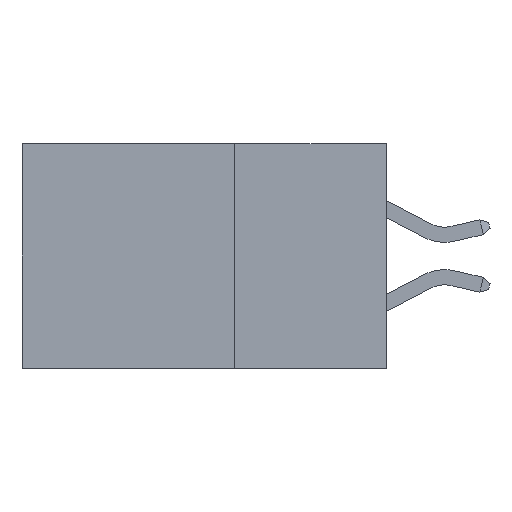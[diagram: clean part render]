
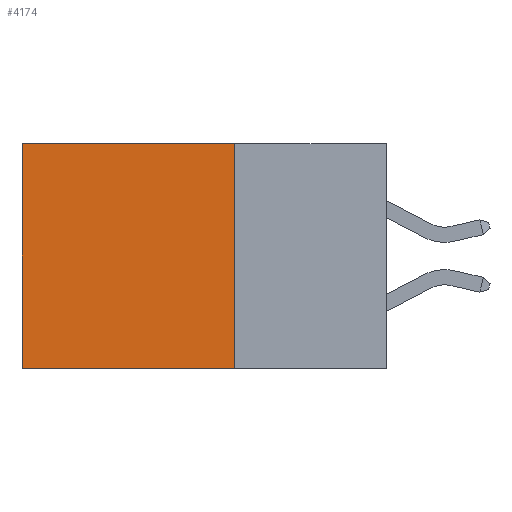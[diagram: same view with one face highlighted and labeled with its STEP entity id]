
A CAD part, left-side view. The second image highlights one B-rep face of the part: STEP entity #4174.
In plain terms, the highlighted planar face has unit normal (-1, 0, 0).
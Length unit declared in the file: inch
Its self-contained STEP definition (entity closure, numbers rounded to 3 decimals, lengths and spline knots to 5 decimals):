
#1862 = DIRECTION ( 'NONE',  ( 0., 0., -1. ) ) ;
#2205 = DIRECTION ( 'NONE',  ( 0., 1., 0. ) ) ;
#2445 = PLANE ( 'NONE',  #5829 ) ;
#2631 = LINE ( 'NONE', #12077, #5681 ) ;
#2814 = DIRECTION ( 'NONE',  ( 0., 0., -1. ) ) ;
#3792 = LINE ( 'NONE', #11962, #10301 ) ;
#4174 = ADVANCED_FACE ( 'NONE', ( #11785 ), #2445, .F. ) ;
#4543 = VECTOR ( 'NONE', #5913, 39.37008 ) ;
#4749 = DIRECTION ( 'NONE',  ( 0., 0., -1. ) ) ;
#5252 = ORIENTED_EDGE ( 'NONE', *, *, #10076, .T. ) ;
#5388 = CARTESIAN_POINT ( 'NONE',  ( 0.298, 0.25, -0.37 ) ) ;
#5681 = VECTOR ( 'NONE', #4749, 39.37008 ) ;
#5691 = LINE ( 'NONE', #14595, #4543 ) ;
#5829 = AXIS2_PLACEMENT_3D ( 'NONE', #8624, #8893, #2814 ) ;
#5913 = DIRECTION ( 'NONE',  ( 0., 1., 0. ) ) ;
#6825 = CARTESIAN_POINT ( 'NONE',  ( 0.298, 0.6, 0. ) ) ;
#7358 = ORIENTED_EDGE ( 'NONE', *, *, #8636, .F. ) ;
#7545 = VERTEX_POINT ( 'NONE', #5388 ) ;
#8370 = EDGE_CURVE ( 'NONE', #7545, #11176, #3792, .T. ) ;
#8624 = CARTESIAN_POINT ( 'NONE',  ( 0.298, 0.25, 0. ) ) ;
#8636 = EDGE_CURVE ( 'NONE', #13488, #7545, #2631, .T. ) ;
#8893 = DIRECTION ( 'NONE',  ( 1., 0., 0. ) ) ;
#9128 = CARTESIAN_POINT ( 'NONE',  ( 0.298, 0.6, 0. ) ) ;
#10076 = EDGE_CURVE ( 'NONE', #14607, #11176, #15576, .T. ) ;
#10301 = VECTOR ( 'NONE', #2205, 39.37008 ) ;
#10863 = CARTESIAN_POINT ( 'NONE',  ( 0.298, 0.25, 0. ) ) ;
#10955 = EDGE_CURVE ( 'NONE', #13488, #14607, #5691, .T. ) ;
#11176 = VERTEX_POINT ( 'NONE', #11348 ) ;
#11348 = CARTESIAN_POINT ( 'NONE',  ( 0.298, 0.6, -0.37 ) ) ;
#11500 = VECTOR ( 'NONE', #1862, 39.37008 ) ;
#11732 = ORIENTED_EDGE ( 'NONE', *, *, #10955, .T. ) ;
#11785 = FACE_OUTER_BOUND ( 'NONE', #15904, .T. ) ;
#11962 = CARTESIAN_POINT ( 'NONE',  ( 0.298, 0.25, -0.37 ) ) ;
#12077 = CARTESIAN_POINT ( 'NONE',  ( 0.298, 0.25, 0. ) ) ;
#12968 = ORIENTED_EDGE ( 'NONE', *, *, #8370, .F. ) ;
#13488 = VERTEX_POINT ( 'NONE', #10863 ) ;
#14595 = CARTESIAN_POINT ( 'NONE',  ( 0.298, 0.25, 0. ) ) ;
#14607 = VERTEX_POINT ( 'NONE', #6825 ) ;
#15576 = LINE ( 'NONE', #9128, #11500 ) ;
#15904 = EDGE_LOOP ( 'NONE', ( #5252, #12968, #7358, #11732 ) ) ;
